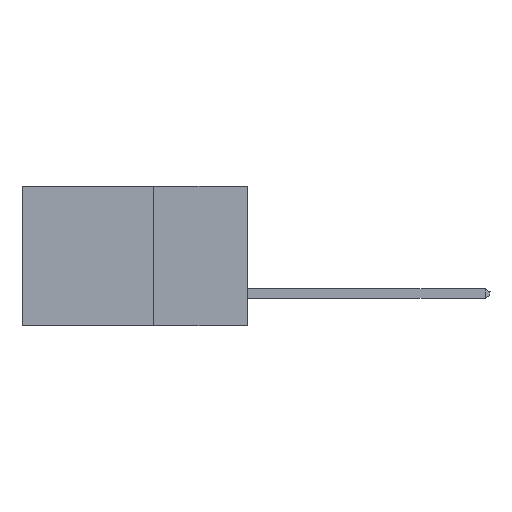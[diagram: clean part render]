
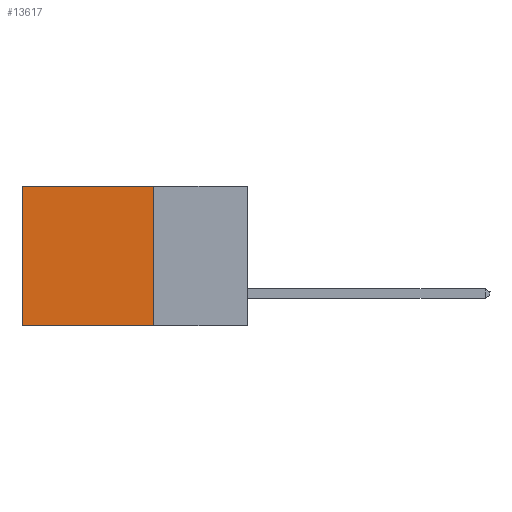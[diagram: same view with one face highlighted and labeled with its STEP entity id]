
A CAD part, left-side view. The second image highlights one B-rep face of the part: STEP entity #13617.
In plain terms, the highlighted planar face has unit normal (-1, 0, 0).
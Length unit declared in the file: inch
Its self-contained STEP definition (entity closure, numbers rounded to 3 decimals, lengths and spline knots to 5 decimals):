
#118 = CARTESIAN_POINT ( 'NONE',  ( 0.2615, 0.25, 0. ) ) ;
#777 = EDGE_CURVE ( 'NONE', #18386, #835, #9982, .T. ) ;
#835 = VERTEX_POINT ( 'NONE', #10174 ) ;
#2596 = EDGE_CURVE ( 'NONE', #5855, #10046, #14481, .T. ) ;
#2726 = VECTOR ( 'NONE', #6010, 39.37008 ) ;
#3041 = VECTOR ( 'NONE', #15956, 39.37008 ) ;
#3457 = CARTESIAN_POINT ( 'NONE',  ( 0.2615, 0.25, -0.37 ) ) ;
#4117 = CARTESIAN_POINT ( 'NONE',  ( 0.2615, 0.6, 0. ) ) ;
#5617 = DIRECTION ( 'NONE',  ( 0., 0., -1. ) ) ;
#5855 = VERTEX_POINT ( 'NONE', #4117 ) ;
#6010 = DIRECTION ( 'NONE',  ( 0., 1., 0. ) ) ;
#6064 = DIRECTION ( 'NONE',  ( 0., 0., -1. ) ) ;
#8277 = VECTOR ( 'NONE', #5617, 39.37008 ) ;
#8527 = ORIENTED_EDGE ( 'NONE', *, *, #777, .F. ) ;
#9482 = CARTESIAN_POINT ( 'NONE',  ( 0.2615, 0.25, -0.37 ) ) ;
#9938 = CARTESIAN_POINT ( 'NONE',  ( 0.2615, 0.25, 0. ) ) ;
#9982 = LINE ( 'NONE', #10079, #3041 ) ;
#10046 = VERTEX_POINT ( 'NONE', #16776 ) ;
#10079 = CARTESIAN_POINT ( 'NONE',  ( 0.2615, 0.25, -0.37 ) ) ;
#10174 = CARTESIAN_POINT ( 'NONE',  ( 0.2615, 0.25, -0.37 ) ) ;
#10537 = EDGE_LOOP ( 'NONE', ( #19357, #11947, #8527, #14001 ) ) ;
#11082 = DIRECTION ( 'NONE',  ( 0., 1., 0. ) ) ;
#11947 = ORIENTED_EDGE ( 'NONE', *, *, #19177, .F. ) ;
#12423 = FACE_OUTER_BOUND ( 'NONE', #10537, .T. ) ;
#13575 = LINE ( 'NONE', #118, #2726 ) ;
#13617 = ADVANCED_FACE ( 'NONE', ( #12423 ), #15223, .F. ) ;
#13865 = LINE ( 'NONE', #9482, #18468 ) ;
#14001 = ORIENTED_EDGE ( 'NONE', *, *, #16590, .T. ) ;
#14481 = LINE ( 'NONE', #16178, #8277 ) ;
#15223 = PLANE ( 'NONE',  #15612 ) ;
#15612 = AXIS2_PLACEMENT_3D ( 'NONE', #3457, #17001, #6064 ) ;
#15956 = DIRECTION ( 'NONE',  ( 0., 0., -1. ) ) ;
#16178 = CARTESIAN_POINT ( 'NONE',  ( 0.2615, 0.6, -0.37 ) ) ;
#16590 = EDGE_CURVE ( 'NONE', #18386, #5855, #13575, .T. ) ;
#16776 = CARTESIAN_POINT ( 'NONE',  ( 0.2615, 0.6, -0.37 ) ) ;
#17001 = DIRECTION ( 'NONE',  ( 1., 0., 0. ) ) ;
#18386 = VERTEX_POINT ( 'NONE', #9938 ) ;
#18468 = VECTOR ( 'NONE', #11082, 39.37008 ) ;
#19177 = EDGE_CURVE ( 'NONE', #835, #10046, #13865, .T. ) ;
#19357 = ORIENTED_EDGE ( 'NONE', *, *, #2596, .T. ) ;
